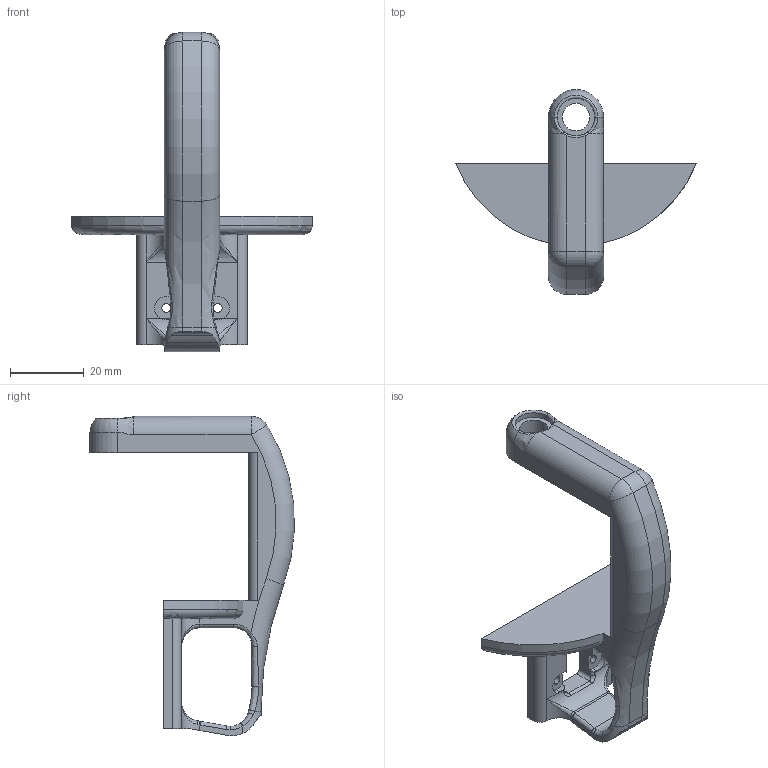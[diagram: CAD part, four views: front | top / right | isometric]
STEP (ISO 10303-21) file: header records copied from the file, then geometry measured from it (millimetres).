
FILE_DESCRIPTION (( 'STEP AP203' ), '1' );
FILE_NAME ('Trigger_Guard.STEP', '2013-11-14T05:08:41', ( '' ), ( '' ), 'SwSTEP 2.0', 'SolidWorks 2013', '' );
FILE_SCHEMA (( 'CONFIG_CONTROL_DESIGN' ));
Length unit declared in the file: millimetre
Products named in the file (1): Trigger_Guard
Bounding box: 65.38 x 55.67 x 86.84 mm (x, y, z)
Volume: 24302.7 mm3; surface area: 10620.3 mm2
Topology: 1 solids, 1 shells, 125 faces, 320 edges, 190 vertices
Faces by surface type: cylinder 51, plane 29, bspline 26, torus 17, sphere 2
Entity records: 4731 total; most frequent: CARTESIAN_POINT 1786, ORIENTED_EDGE 632, DIRECTION 586, EDGE_CURVE 316, AXIS2_PLACEMENT_3D 236, VERTEX_POINT 190, CIRCLE 136, EDGE_LOOP 132
